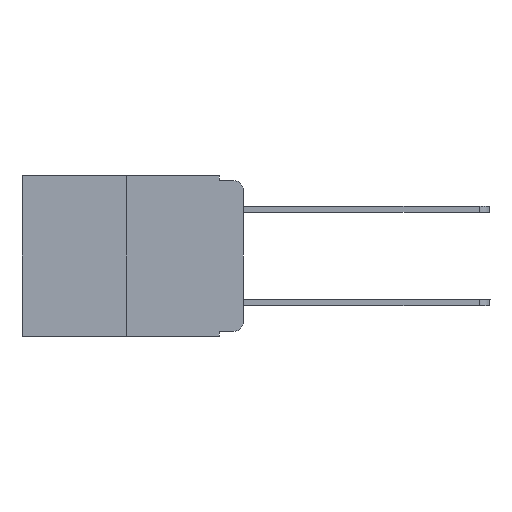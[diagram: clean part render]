
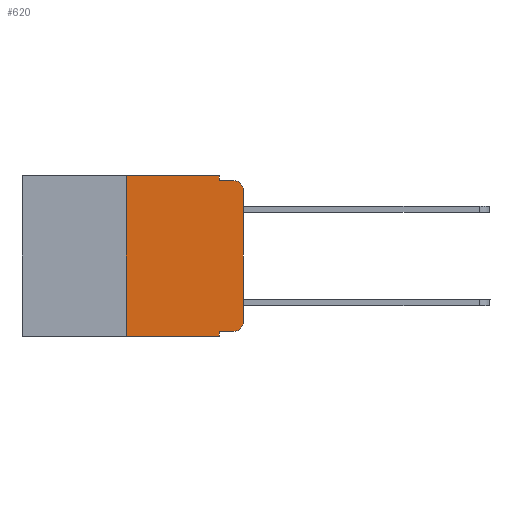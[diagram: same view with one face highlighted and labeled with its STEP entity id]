
A CAD part, left-side view. The second image highlights one B-rep face of the part: STEP entity #620.
In plain terms, the highlighted planar face has unit normal (-1, 0, 0).
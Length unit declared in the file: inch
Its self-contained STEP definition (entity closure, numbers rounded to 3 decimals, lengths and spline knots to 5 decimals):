
#20 = CARTESIAN_POINT ( 'NONE',  ( 0., 0., 0. ) ) ;
#276 = LINE ( 'NONE', #6243, #8324 ) ;
#331 = ORIENTED_EDGE ( 'NONE', *, *, #4291, .T. ) ;
#385 = ORIENTED_EDGE ( 'NONE', *, *, #4660, .F. ) ;
#461 = DIRECTION ( 'NONE',  ( 0., 0., -1. ) ) ;
#620 = ADVANCED_FACE ( 'NONE', ( #2987 ), #6540, .F. ) ;
#664 = LINE ( 'NONE', #5225, #2140 ) ;
#749 = VERTEX_POINT ( 'NONE', #2029 ) ;
#801 = VERTEX_POINT ( 'NONE', #3855 ) ;
#1076 = VERTEX_POINT ( 'NONE', #6917 ) ;
#1141 = ORIENTED_EDGE ( 'NONE', *, *, #1607, .F. ) ;
#1426 = CARTESIAN_POINT ( 'NONE',  ( 0., 0.25, 0. ) ) ;
#1471 = LINE ( 'NONE', #8370, #3752 ) ;
#1607 = EDGE_CURVE ( 'NONE', #1076, #801, #8940, .T. ) ;
#2029 = CARTESIAN_POINT ( 'NONE',  ( 0., 0.02, -0.333 ) ) ;
#2140 = VECTOR ( 'NONE', #6716, 39.37008 ) ;
#2228 = ORIENTED_EDGE ( 'NONE', *, *, #8986, .T. ) ;
#2379 = CARTESIAN_POINT ( 'NONE',  ( 0., 0.02, -0.01 ) ) ;
#2405 = LINE ( 'NONE', #7003, #3426 ) ;
#2665 = CIRCLE ( 'NONE', #5179, 0.02 ) ;
#2669 = DIRECTION ( 'NONE',  ( 0., -1., 0. ) ) ;
#2950 = ORIENTED_EDGE ( 'NONE', *, *, #3989, .F. ) ;
#2966 = CIRCLE ( 'NONE', #7227, 0.02 ) ;
#2987 = FACE_OUTER_BOUND ( 'NONE', #5625, .T. ) ;
#3426 = VECTOR ( 'NONE', #5421, 39.37008 ) ;
#3427 = VERTEX_POINT ( 'NONE', #6519 ) ;
#3718 = DIRECTION ( 'NONE',  ( 0., -1., 0. ) ) ;
#3752 = VECTOR ( 'NONE', #3718, 39.37008 ) ;
#3836 = EDGE_CURVE ( 'NONE', #6006, #3427, #5952, .T. ) ;
#3855 = CARTESIAN_POINT ( 'NONE',  ( 0., 0.051, -0.01 ) ) ;
#3989 = EDGE_CURVE ( 'NONE', #8807, #6146, #276, .T. ) ;
#4024 = DIRECTION ( 'NONE',  ( 0., 0., 1. ) ) ;
#4068 = EDGE_CURVE ( 'NONE', #749, #6006, #2966, .T. ) ;
#4123 = CARTESIAN_POINT ( 'NONE',  ( 0., 0.02, -0.03 ) ) ;
#4291 = EDGE_CURVE ( 'NONE', #8807, #5719, #1471, .T. ) ;
#4342 = CARTESIAN_POINT ( 'NONE',  ( 0., 0.051, 0. ) ) ;
#4660 = EDGE_CURVE ( 'NONE', #6146, #1076, #664, .T. ) ;
#4775 = EDGE_CURVE ( 'NONE', #801, #6191, #2405, .T. ) ;
#4819 = DIRECTION ( 'NONE',  ( -1., 0., 0. ) ) ;
#4913 = ORIENTED_EDGE ( 'NONE', *, *, #4068, .T. ) ;
#5012 = VECTOR ( 'NONE', #9410, 39.37008 ) ;
#5179 = AXIS2_PLACEMENT_3D ( 'NONE', #4123, #7130, #461 ) ;
#5225 = CARTESIAN_POINT ( 'NONE',  ( 0., 0.473, 0. ) ) ;
#5420 = EDGE_CURVE ( 'NONE', #7678, #5719, #5604, .T. ) ;
#5421 = DIRECTION ( 'NONE',  ( 0., -1., 0. ) ) ;
#5555 = CARTESIAN_POINT ( 'NONE',  ( 0., 0., -0.313 ) ) ;
#5604 = LINE ( 'NONE', #8619, #5012 ) ;
#5625 = EDGE_LOOP ( 'NONE', ( #5691, #2228, #5748, #1141, #385, #2950, #331, #7180, #7600, #4913 ) ) ;
#5691 = ORIENTED_EDGE ( 'NONE', *, *, #3836, .T. ) ;
#5719 = VERTEX_POINT ( 'NONE', #7332 ) ;
#5732 = VECTOR ( 'NONE', #6149, 39.37008 ) ;
#5748 = ORIENTED_EDGE ( 'NONE', *, *, #4775, .F. ) ;
#5847 = DIRECTION ( 'NONE',  ( 1., 0., 0. ) ) ;
#5952 = LINE ( 'NONE', #20, #5732 ) ;
#6006 = VERTEX_POINT ( 'NONE', #5555 ) ;
#6146 = VERTEX_POINT ( 'NONE', #1426 ) ;
#6149 = DIRECTION ( 'NONE',  ( 0., 0., 1. ) ) ;
#6191 = VERTEX_POINT ( 'NONE', #2379 ) ;
#6243 = CARTESIAN_POINT ( 'NONE',  ( 0., 0.25, 0. ) ) ;
#6354 = LINE ( 'NONE', #7152, #8327 ) ;
#6439 = CARTESIAN_POINT ( 'NONE',  ( 0., 0.051, -0.333 ) ) ;
#6519 = CARTESIAN_POINT ( 'NONE',  ( 0., 0., -0.03 ) ) ;
#6540 = PLANE ( 'NONE',  #7642 ) ;
#6641 = DIRECTION ( 'NONE',  ( 0., 0., -1. ) ) ;
#6716 = DIRECTION ( 'NONE',  ( 0., -1., 0. ) ) ;
#6917 = CARTESIAN_POINT ( 'NONE',  ( 0., 0.051, 0. ) ) ;
#7003 = CARTESIAN_POINT ( 'NONE',  ( 0., 0.051, -0.01 ) ) ;
#7093 = DIRECTION ( 'NONE',  ( 0., 0., -1. ) ) ;
#7130 = DIRECTION ( 'NONE',  ( -1., 0., 0. ) ) ;
#7152 = CARTESIAN_POINT ( 'NONE',  ( 0., 0.051, -0.333 ) ) ;
#7180 = ORIENTED_EDGE ( 'NONE', *, *, #5420, .F. ) ;
#7227 = AXIS2_PLACEMENT_3D ( 'NONE', #8574, #4819, #7093 ) ;
#7313 = DIRECTION ( 'NONE',  ( 0., 0., -1. ) ) ;
#7332 = CARTESIAN_POINT ( 'NONE',  ( 0., 0.051, -0.343 ) ) ;
#7600 = ORIENTED_EDGE ( 'NONE', *, *, #8572, .T. ) ;
#7642 = AXIS2_PLACEMENT_3D ( 'NONE', #8953, #5847, #6641 ) ;
#7678 = VERTEX_POINT ( 'NONE', #6439 ) ;
#8324 = VECTOR ( 'NONE', #4024, 39.37008 ) ;
#8327 = VECTOR ( 'NONE', #2669, 39.37008 ) ;
#8370 = CARTESIAN_POINT ( 'NONE',  ( 0., 0.473, -0.343 ) ) ;
#8561 = CARTESIAN_POINT ( 'NONE',  ( 0., 0.25, -0.343 ) ) ;
#8572 = EDGE_CURVE ( 'NONE', #7678, #749, #6354, .T. ) ;
#8574 = CARTESIAN_POINT ( 'NONE',  ( 0., 0.02, -0.313 ) ) ;
#8619 = CARTESIAN_POINT ( 'NONE',  ( 0., 0.051, 0. ) ) ;
#8807 = VERTEX_POINT ( 'NONE', #8561 ) ;
#8940 = LINE ( 'NONE', #4342, #9191 ) ;
#8953 = CARTESIAN_POINT ( 'NONE',  ( 0., 0.473, 0. ) ) ;
#8986 = EDGE_CURVE ( 'NONE', #3427, #6191, #2665, .T. ) ;
#9191 = VECTOR ( 'NONE', #7313, 39.37008 ) ;
#9410 = DIRECTION ( 'NONE',  ( 0., 0., -1. ) ) ;
